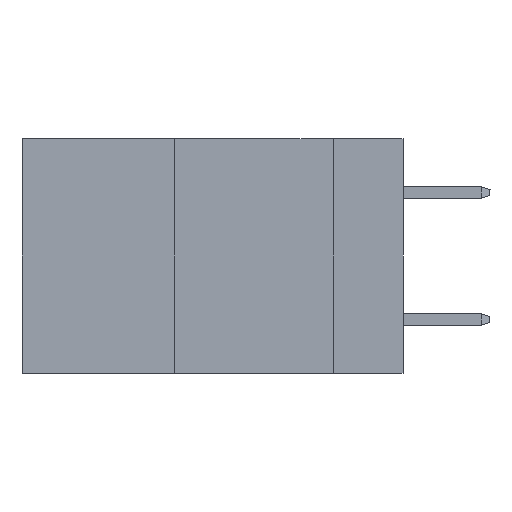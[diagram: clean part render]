
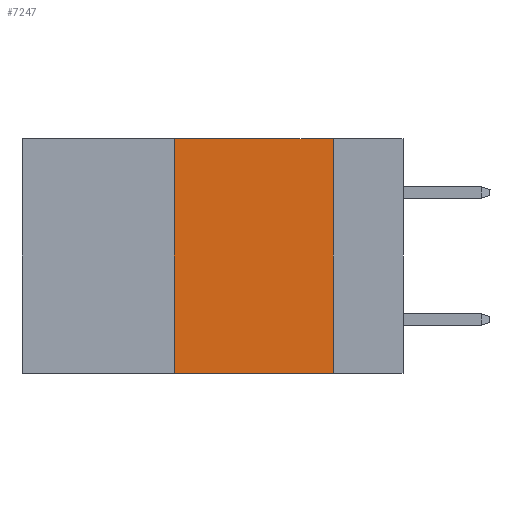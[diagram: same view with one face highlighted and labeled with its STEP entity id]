
A CAD part, left-side view. The second image highlights one B-rep face of the part: STEP entity #7247.
In plain terms, the highlighted planar face has unit normal (-1, 0, 0).
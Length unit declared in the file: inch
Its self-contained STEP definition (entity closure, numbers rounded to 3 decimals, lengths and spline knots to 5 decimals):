
#817 = CARTESIAN_POINT ( 'NONE',  ( 0., 0.36, 0. ) ) ;
#1524 = AXIS2_PLACEMENT_3D ( 'NONE', #12916, #4760, #8144 ) ;
#1882 = VERTEX_POINT ( 'NONE', #7233 ) ;
#1936 = CARTESIAN_POINT ( 'NONE',  ( 0., 0.6, 0. ) ) ;
#2766 = EDGE_CURVE ( 'NONE', #5094, #3618, #17667, .T. ) ;
#3174 = VERTEX_POINT ( 'NONE', #13228 ) ;
#3569 = CARTESIAN_POINT ( 'NONE',  ( 0., 0.6, -0.37 ) ) ;
#3618 = VERTEX_POINT ( 'NONE', #16242 ) ;
#4760 = DIRECTION ( 'NONE',  ( 1., 0., 0. ) ) ;
#5094 = VERTEX_POINT ( 'NONE', #18326 ) ;
#7151 = DIRECTION ( 'NONE',  ( 0., 0., 1. ) ) ;
#7233 = CARTESIAN_POINT ( 'NONE',  ( 0., 0.36, 0. ) ) ;
#7247 = ADVANCED_FACE ( 'NONE', ( #17238 ), #7937, .F. ) ;
#7937 = PLANE ( 'NONE',  #1524 ) ;
#8144 = DIRECTION ( 'NONE',  ( 0., 0., -1. ) ) ;
#9069 = EDGE_LOOP ( 'NONE', ( #20017, #17724, #14749, #13090 ) ) ;
#9160 = CARTESIAN_POINT ( 'NONE',  ( 0., 0.11, 0. ) ) ;
#9777 = VECTOR ( 'NONE', #15391, 39.37008 ) ;
#10601 = EDGE_CURVE ( 'NONE', #1882, #3174, #12515, .T. ) ;
#11776 = VECTOR ( 'NONE', #16112, 39.37008 ) ;
#12513 = LINE ( 'NONE', #9160, #9777 ) ;
#12515 = LINE ( 'NONE', #1936, #13139 ) ;
#12916 = CARTESIAN_POINT ( 'NONE',  ( 0., 0.6, 0. ) ) ;
#12969 = LINE ( 'NONE', #817, #13472 ) ;
#13090 = ORIENTED_EDGE ( 'NONE', *, *, #2766, .T. ) ;
#13139 = VECTOR ( 'NONE', #14068, 39.37008 ) ;
#13228 = CARTESIAN_POINT ( 'NONE',  ( 0., 0.11, 0. ) ) ;
#13472 = VECTOR ( 'NONE', #7151, 39.37008 ) ;
#13803 = EDGE_CURVE ( 'NONE', #5094, #1882, #12969, .T. ) ;
#14068 = DIRECTION ( 'NONE',  ( 0., -1., 0. ) ) ;
#14749 = ORIENTED_EDGE ( 'NONE', *, *, #13803, .F. ) ;
#15391 = DIRECTION ( 'NONE',  ( 0., 0., -1. ) ) ;
#16112 = DIRECTION ( 'NONE',  ( 0., -1., 0. ) ) ;
#16242 = CARTESIAN_POINT ( 'NONE',  ( 0., 0.11, -0.37 ) ) ;
#17238 = FACE_OUTER_BOUND ( 'NONE', #9069, .T. ) ;
#17667 = LINE ( 'NONE', #3569, #11776 ) ;
#17724 = ORIENTED_EDGE ( 'NONE', *, *, #10601, .F. ) ;
#18326 = CARTESIAN_POINT ( 'NONE',  ( 0., 0.36, -0.37 ) ) ;
#19564 = EDGE_CURVE ( 'NONE', #3174, #3618, #12513, .T. ) ;
#20017 = ORIENTED_EDGE ( 'NONE', *, *, #19564, .F. ) ;
